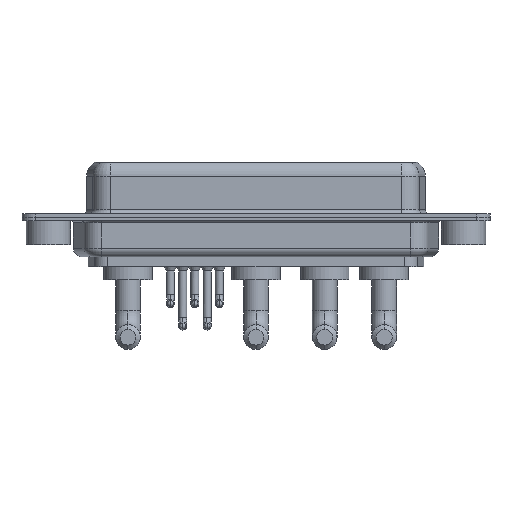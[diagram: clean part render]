
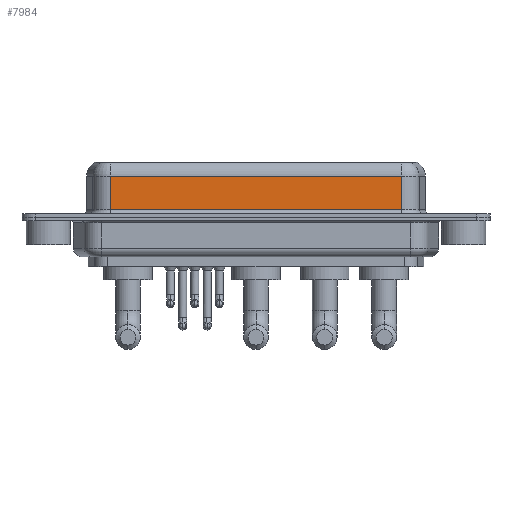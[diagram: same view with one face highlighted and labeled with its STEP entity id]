
A CAD part, front view. The second image highlights one B-rep face of the part: STEP entity #7984.
In plain terms, the highlighted planar face has unit normal (0, -1, 0).
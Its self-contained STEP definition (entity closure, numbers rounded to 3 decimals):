
#295 = VECTOR ( 'NONE', #7136, 1000. ) ;
#1014 = CARTESIAN_POINT ( 'NONE',  ( 7.013, -3.95, 0.9 ) ) ;
#1407 = VECTOR ( 'NONE', #8792, 1000. ) ;
#2236 = CARTESIAN_POINT ( 'NONE',  ( 7.013, -3.95, 4.65 ) ) ;
#2350 = CARTESIAN_POINT ( 'NONE',  ( 7.013, -3.95, 6.4 ) ) ;
#2666 = CARTESIAN_POINT ( 'NONE',  ( 40.037, -3.95, 6.4 ) ) ;
#4075 = EDGE_CURVE ( 'NONE', #6826, #8060, #7131, .T. ) ;
#4544 = LINE ( 'NONE', #16144, #295 ) ;
#4743 = ORIENTED_EDGE ( 'NONE', *, *, #14694, .T. ) ;
#5389 = VERTEX_POINT ( 'NONE', #11173 ) ;
#5448 = AXIS2_PLACEMENT_3D ( 'NONE', #15559, #15826, #11729 ) ;
#5497 = CARTESIAN_POINT ( 'NONE',  ( 40.037, -3.95, 4.65 ) ) ;
#6783 = EDGE_CURVE ( 'NONE', #10023, #5389, #4544, .T. ) ;
#6823 = LINE ( 'NONE', #2666, #15639 ) ;
#6826 = VERTEX_POINT ( 'NONE', #5497 ) ;
#7131 = LINE ( 'NONE', #9502, #1407 ) ;
#7136 = DIRECTION ( 'NONE',  ( 1., 0., 0. ) ) ;
#7984 = ADVANCED_FACE ( 'NONE', ( #14431 ), #10223, .F. ) ;
#8060 = VERTEX_POINT ( 'NONE', #2236 ) ;
#8207 = EDGE_CURVE ( 'NONE', #6826, #5389, #6823, .T. ) ;
#8792 = DIRECTION ( 'NONE',  ( -1., 0., 0. ) ) ;
#8825 = ORIENTED_EDGE ( 'NONE', *, *, #4075, .T. ) ;
#9017 = EDGE_LOOP ( 'NONE', ( #14392, #8825, #4743, #11634 ) ) ;
#9502 = CARTESIAN_POINT ( 'NONE',  ( 40.037, -3.95, 4.65 ) ) ;
#10023 = VERTEX_POINT ( 'NONE', #1014 ) ;
#10223 = PLANE ( 'NONE',  #5448 ) ;
#11003 = VECTOR ( 'NONE', #12973, 1000. ) ;
#11173 = CARTESIAN_POINT ( 'NONE',  ( 40.037, -3.95, 0.9 ) ) ;
#11634 = ORIENTED_EDGE ( 'NONE', *, *, #6783, .T. ) ;
#11729 = DIRECTION ( 'NONE',  ( 0., 0., 1. ) ) ;
#12973 = DIRECTION ( 'NONE',  ( 0., 0., -1. ) ) ;
#14284 = LINE ( 'NONE', #2350, #11003 ) ;
#14392 = ORIENTED_EDGE ( 'NONE', *, *, #8207, .F. ) ;
#14431 = FACE_OUTER_BOUND ( 'NONE', #9017, .T. ) ;
#14694 = EDGE_CURVE ( 'NONE', #8060, #10023, #14284, .T. ) ;
#15559 = CARTESIAN_POINT ( 'NONE',  ( 40.037, -3.95, 6.4 ) ) ;
#15639 = VECTOR ( 'NONE', #16170, 1000. ) ;
#15826 = DIRECTION ( 'NONE',  ( 0., 1., 0. ) ) ;
#16144 = CARTESIAN_POINT ( 'NONE',  ( 40.037, -3.95, 0.9 ) ) ;
#16170 = DIRECTION ( 'NONE',  ( 0., 0., -1. ) ) ;
